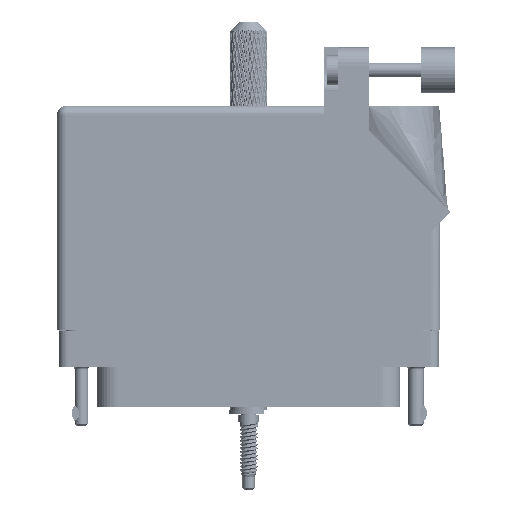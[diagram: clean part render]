
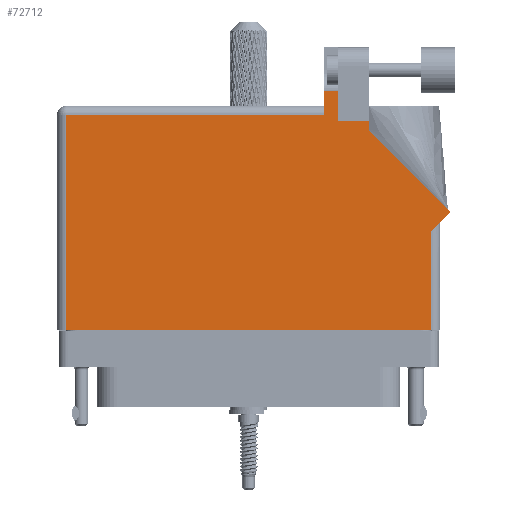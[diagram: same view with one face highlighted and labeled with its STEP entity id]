
A CAD part, front view. The second image highlights one B-rep face of the part: STEP entity #72712.
In plain terms, the highlighted face is planar.
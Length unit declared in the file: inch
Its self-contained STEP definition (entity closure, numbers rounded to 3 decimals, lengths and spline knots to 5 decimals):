
#62 = LINE ( 'NONE', #121750, #23025 ) ;
#94 = DIRECTION ( 'NONE',  ( 0., 0., -1. ) ) ;
#524 = ORIENTED_EDGE ( 'NONE', *, *, #51441, .T. ) ;
#1066 = ORIENTED_EDGE ( 'NONE', *, *, #15873, .T. ) ;
#1374 = CARTESIAN_POINT ( 'NONE',  ( -1.306, 1.43, 0.455 ) ) ;
#1640 = VERTEX_POINT ( 'NONE', #77597 ) ;
#4197 = ORIENTED_EDGE ( 'NONE', *, *, #6338, .T. ) ;
#5115 = DIRECTION ( 'NONE',  ( -0.707, 0.707, 0. ) ) ;
#6162 = VERTEX_POINT ( 'NONE', #59660 ) ;
#6286 = CARTESIAN_POINT ( 'NONE',  ( 0.513, 1.43, 0.455 ) ) ;
#6338 = EDGE_CURVE ( 'NONE', #112026, #90691, #67684, .T. ) ;
#7363 = VECTOR ( 'NONE', #36496, 39.37008 ) ;
#8608 = EDGE_CURVE ( 'NONE', #6162, #126161, #59659, .T. ) ;
#12197 = VECTOR ( 'NONE', #64760, 39.37008 ) ;
#12519 = EDGE_LOOP ( 'NONE', ( #109656, #97150, #524, #100446, #1066, #4197, #102975, #83392, #73072, #22843, #28909 ) ) ;
#14427 = EDGE_CURVE ( 'NONE', #34278, #77299, #77093, .T. ) ;
#14964 = FACE_OUTER_BOUND ( 'NONE', #12519, .T. ) ;
#15770 = CARTESIAN_POINT ( 'NONE',  ( 0.82, 1.26442, 0.455 ) ) ;
#15873 = EDGE_CURVE ( 'NONE', #77299, #112026, #62, .T. ) ;
#16524 = VERTEX_POINT ( 'NONE', #125909 ) ;
#18484 = LINE ( 'NONE', #79935, #58468 ) ;
#18711 = CARTESIAN_POINT ( 'NONE',  ( -1.244, 1.368, 0.455 ) ) ;
#19161 = CARTESIAN_POINT ( 'NONE',  ( 0.513, 1.5315, 0.455 ) ) ;
#20233 = PLANE ( 'NONE',  #34211 ) ;
#22843 = ORIENTED_EDGE ( 'NONE', *, *, #56651, .T. ) ;
#23025 = VECTOR ( 'NONE', #86634, 39.37008 ) ;
#24271 = DIRECTION ( 'NONE',  ( 0., -1., 0. ) ) ;
#24554 = CARTESIAN_POINT ( 'NONE',  ( 0.607, 1.33, 0.455 ) ) ;
#24765 = CARTESIAN_POINT ( 'NONE',  ( -1.306, -0.1, 0.455 ) ) ;
#26208 = CARTESIAN_POINT ( 'NONE',  ( 0.93777, 1.5315, 0.455 ) ) ;
#27820 = VECTOR ( 'NONE', #58766, 39.37008 ) ;
#28909 = ORIENTED_EDGE ( 'NONE', *, *, #8608, .T. ) ;
#34211 = AXIS2_PLACEMENT_3D ( 'NONE', #1374, #94, #88961 ) ;
#34278 = VERTEX_POINT ( 'NONE', #47790 ) ;
#34632 = CARTESIAN_POINT ( 'NONE',  ( 1.37671, 0.70771, 0.455 ) ) ;
#35025 = EDGE_CURVE ( 'NONE', #90691, #90023, #103502, .T. ) ;
#36496 = DIRECTION ( 'NONE',  ( -1., 0., 0. ) ) ;
#37602 = VECTOR ( 'NONE', #116373, 39.37008 ) ;
#39677 = VECTOR ( 'NONE', #50267, 39.37008 ) ;
#42473 = LINE ( 'NONE', #34632, #50277 ) ;
#42638 = LINE ( 'NONE', #26208, #7363 ) ;
#43699 = EDGE_CURVE ( 'NONE', #126161, #16524, #108247, .T. ) ;
#44457 = CARTESIAN_POINT ( 'NONE',  ( 1.244, 0.575, 0.455 ) ) ;
#45964 = EDGE_CURVE ( 'NONE', #90023, #1640, #18484, .T. ) ;
#47790 = CARTESIAN_POINT ( 'NONE',  ( 0.513, 1.368, 0.455 ) ) ;
#47800 = VERTEX_POINT ( 'NONE', #120180 ) ;
#50267 = DIRECTION ( 'NONE',  ( -1., 0., 0. ) ) ;
#50277 = VECTOR ( 'NONE', #5115, 39.37008 ) ;
#51243 = VECTOR ( 'NONE', #104170, 39.37008 ) ;
#51441 = EDGE_CURVE ( 'NONE', #53067, #34278, #79066, .T. ) ;
#52869 = VECTOR ( 'NONE', #24271, 39.37008 ) ;
#53067 = VERTEX_POINT ( 'NONE', #19161 ) ;
#56651 = EDGE_CURVE ( 'NONE', #47800, #6162, #105914, .T. ) ;
#58468 = VECTOR ( 'NONE', #70016, 39.37008 ) ;
#58766 = DIRECTION ( 'NONE',  ( -1., 0., 0. ) ) ;
#59659 = LINE ( 'NONE', #88157, #39677 ) ;
#59660 = CARTESIAN_POINT ( 'NONE',  ( 0.82, 1.33, 0.455 ) ) ;
#64760 = DIRECTION ( 'NONE',  ( 0., 1., 0. ) ) ;
#67684 = LINE ( 'NONE', #24765, #75420 ) ;
#70016 = DIRECTION ( 'NONE',  ( 0.707, 0.707, 0. ) ) ;
#72712 = ADVANCED_FACE ( 'NONE', ( #14964 ), #20233, .F. ) ;
#73072 = ORIENTED_EDGE ( 'NONE', *, *, #122503, .T. ) ;
#75420 = VECTOR ( 'NONE', #124302, 39.37008 ) ;
#77093 = LINE ( 'NONE', #77708, #27820 ) ;
#77211 = CARTESIAN_POINT ( 'NONE',  ( -1.244, -0.1, 0.455 ) ) ;
#77299 = VERTEX_POINT ( 'NONE', #18711 ) ;
#77597 = CARTESIAN_POINT ( 'NONE',  ( 1.37671, 0.70771, 0.455 ) ) ;
#77708 = CARTESIAN_POINT ( 'NONE',  ( -1.306, 1.368, 0.455 ) ) ;
#79066 = LINE ( 'NONE', #6286, #52869 ) ;
#79935 = CARTESIAN_POINT ( 'NONE',  ( 1.306, 0.637, 0.455 ) ) ;
#83392 = ORIENTED_EDGE ( 'NONE', *, *, #45964, .T. ) ;
#86634 = DIRECTION ( 'NONE',  ( 0., -1., 0. ) ) ;
#88157 = CARTESIAN_POINT ( 'NONE',  ( 0.82, 1.33, 0.455 ) ) ;
#88961 = DIRECTION ( 'NONE',  ( -1., 0., 0. ) ) ;
#90023 = VERTEX_POINT ( 'NONE', #44457 ) ;
#90691 = VERTEX_POINT ( 'NONE', #114219 ) ;
#97150 = ORIENTED_EDGE ( 'NONE', *, *, #116254, .T. ) ;
#100446 = ORIENTED_EDGE ( 'NONE', *, *, #14427, .T. ) ;
#102975 = ORIENTED_EDGE ( 'NONE', *, *, #35025, .T. ) ;
#103502 = LINE ( 'NONE', #123030, #51243 ) ;
#104170 = DIRECTION ( 'NONE',  ( 0., 1., 0. ) ) ;
#105914 = LINE ( 'NONE', #15770, #12197 ) ;
#106585 = CARTESIAN_POINT ( 'NONE',  ( 0.607, 1.33, 0.455 ) ) ;
#108247 = LINE ( 'NONE', #106585, #37602 ) ;
#109656 = ORIENTED_EDGE ( 'NONE', *, *, #43699, .T. ) ;
#112026 = VERTEX_POINT ( 'NONE', #77211 ) ;
#114219 = CARTESIAN_POINT ( 'NONE',  ( 1.244, -0.1, 0.455 ) ) ;
#116254 = EDGE_CURVE ( 'NONE', #16524, #53067, #42638, .T. ) ;
#116373 = DIRECTION ( 'NONE',  ( 0., 1., 0. ) ) ;
#120180 = CARTESIAN_POINT ( 'NONE',  ( 0.82, 1.26442, 0.455 ) ) ;
#121750 = CARTESIAN_POINT ( 'NONE',  ( -1.244, -0.1, 0.455 ) ) ;
#122503 = EDGE_CURVE ( 'NONE', #1640, #47800, #42473, .T. ) ;
#123030 = CARTESIAN_POINT ( 'NONE',  ( 1.244, 0.637, 0.455 ) ) ;
#124302 = DIRECTION ( 'NONE',  ( 1., 0., 0. ) ) ;
#125909 = CARTESIAN_POINT ( 'NONE',  ( 0.607, 1.5315, 0.455 ) ) ;
#126161 = VERTEX_POINT ( 'NONE', #24554 ) ;
